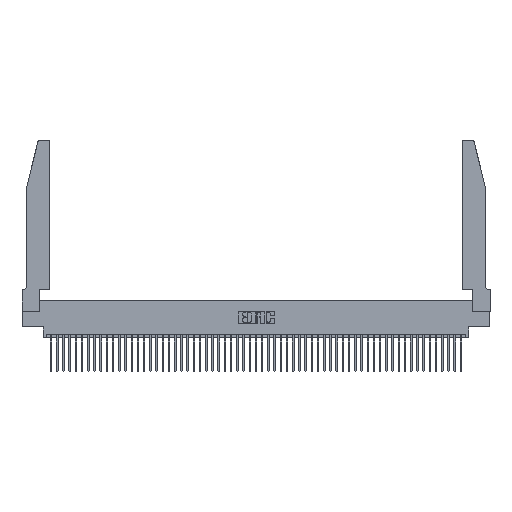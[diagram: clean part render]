
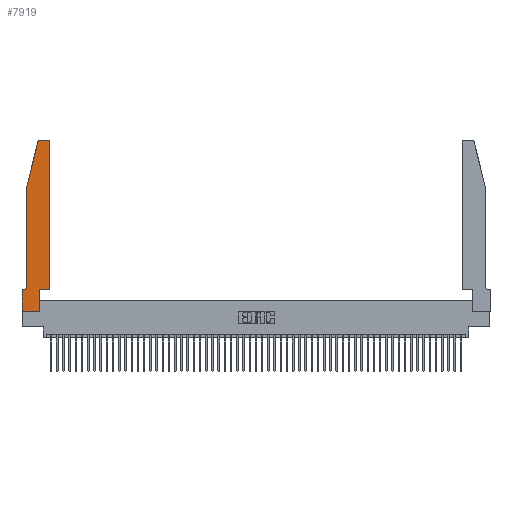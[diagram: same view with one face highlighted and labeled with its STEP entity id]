
A CAD part, top view. The second image highlights one B-rep face of the part: STEP entity #7919.
In plain terms, the highlighted planar face has unit normal (0, 0, 1).
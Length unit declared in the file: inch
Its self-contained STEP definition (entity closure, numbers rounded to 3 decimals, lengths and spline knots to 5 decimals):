
#360 = ORIENTED_EDGE ( 'NONE', *, *, #6956, .T. ) ;
#492 = LINE ( 'NONE', #938, #43675 ) ;
#749 = DIRECTION ( 'NONE',  ( 0., 1., 0. ) ) ;
#938 = CARTESIAN_POINT ( 'NONE',  ( 0.4505, 0.35, 0.37 ) ) ;
#2590 = VECTOR ( 'NONE', #33502, 39.37008 ) ;
#2646 = FACE_OUTER_BOUND ( 'NONE', #4504, .T. ) ;
#3522 = CARTESIAN_POINT ( 'NONE',  ( 0.4205, 2.72, 0.37 ) ) ;
#4024 = DIRECTION ( 'NONE',  ( 0., -1., 0. ) ) ;
#4266 = CARTESIAN_POINT ( 'NONE',  ( 0.0755, 2., 0.37 ) ) ;
#4504 = EDGE_LOOP ( 'NONE', ( #35077, #20084, #11923, #39261, #52693, #35816, #17316, #6054, #360, #19127, #7590, #7361 ) ) ;
#4527 = AXIS2_PLACEMENT_3D ( 'NONE', #27566, #18993, #14943 ) ;
#6054 = ORIENTED_EDGE ( 'NONE', *, *, #8216, .T. ) ;
#6956 = EDGE_CURVE ( 'NONE', #44923, #27076, #21676, .T. ) ;
#7361 = ORIENTED_EDGE ( 'NONE', *, *, #12692, .T. ) ;
#7590 = ORIENTED_EDGE ( 'NONE', *, *, #42156, .T. ) ;
#7919 = ADVANCED_FACE ( 'NONE', ( #2646 ), #35439, .T. ) ;
#8216 = EDGE_CURVE ( 'NONE', #14412, #44923, #12428, .T. ) ;
#8494 = AXIS2_PLACEMENT_3D ( 'NONE', #46907, #8901, #30279 ) ;
#8698 = EDGE_CURVE ( 'NONE', #38435, #44221, #52950, .T. ) ;
#8901 = DIRECTION ( 'NONE',  ( 0., 0., 1. ) ) ;
#11461 = AXIS2_PLACEMENT_3D ( 'NONE', #39875, #18502, #51946 ) ;
#11923 = ORIENTED_EDGE ( 'NONE', *, *, #40419, .T. ) ;
#12428 = LINE ( 'NONE', #50347, #18978 ) ;
#12692 = EDGE_CURVE ( 'NONE', #14862, #17868, #29641, .T. ) ;
#12860 = CARTESIAN_POINT ( 'NONE',  ( 0.2865, 0.35, 0.37 ) ) ;
#14412 = VERTEX_POINT ( 'NONE', #22463 ) ;
#14862 = VERTEX_POINT ( 'NONE', #32825 ) ;
#14943 = DIRECTION ( 'NONE',  ( 1., 0., 0. ) ) ;
#15869 = CARTESIAN_POINT ( 'NONE',  ( 0.0055, 0.35, 0.37 ) ) ;
#16109 = LINE ( 'NONE', #19877, #52101 ) ;
#16722 = CARTESIAN_POINT ( 'NONE',  ( 0.0755, 2., 0.37 ) ) ;
#16853 = DIRECTION ( 'NONE',  ( -1., 0., 0. ) ) ;
#17316 = ORIENTED_EDGE ( 'NONE', *, *, #19793, .T. ) ;
#17868 = VERTEX_POINT ( 'NONE', #32746 ) ;
#18502 = DIRECTION ( 'NONE',  ( 0., 0., -1. ) ) ;
#18978 = VECTOR ( 'NONE', #38453, 39.37008 ) ;
#18993 = DIRECTION ( 'NONE',  ( 0., 0., 1. ) ) ;
#19051 = LINE ( 'NONE', #16722, #51722 ) ;
#19127 = ORIENTED_EDGE ( 'NONE', *, *, #34220, .T. ) ;
#19492 = CARTESIAN_POINT ( 'NONE',  ( 0.4505, 0.35, 0.37 ) ) ;
#19793 = EDGE_CURVE ( 'NONE', #44221, #14412, #50299, .T. ) ;
#19877 = CARTESIAN_POINT ( 'NONE',  ( 0.0755, 2., 0.37 ) ) ;
#20020 = LINE ( 'NONE', #41062, #24580 ) ;
#20084 = ORIENTED_EDGE ( 'NONE', *, *, #39871, .T. ) ;
#20413 = CARTESIAN_POINT ( 'NONE',  ( 0.2865, 0., 0.37 ) ) ;
#21200 = EDGE_CURVE ( 'NONE', #29954, #33107, #16109, .T. ) ;
#21676 = LINE ( 'NONE', #23355, #43976 ) ;
#21954 = VERTEX_POINT ( 'NONE', #28569 ) ;
#22085 = EDGE_CURVE ( 'NONE', #17868, #21954, #35649, .T. ) ;
#22463 = CARTESIAN_POINT ( 'NONE',  ( 0., 0., 0.37 ) ) ;
#23355 = CARTESIAN_POINT ( 'NONE',  ( 0.2865, 0.35, 0.37 ) ) ;
#24565 = CARTESIAN_POINT ( 'NONE',  ( 0., 0.35, 0.37 ) ) ;
#24580 = VECTOR ( 'NONE', #29187, 39.37008 ) ;
#27076 = VERTEX_POINT ( 'NONE', #12860 ) ;
#27566 = CARTESIAN_POINT ( 'NONE',  ( 0., 0.35, 0.37 ) ) ;
#28569 = CARTESIAN_POINT ( 'NONE',  ( 0.284, 2.75, 0.37 ) ) ;
#28717 = CARTESIAN_POINT ( 'NONE',  ( 0.25487, 2.72718, 0.37 ) ) ;
#28938 = CARTESIAN_POINT ( 'NONE',  ( 0.0755, 0.42, 0.37 ) ) ;
#29187 = DIRECTION ( 'NONE',  ( 1., 0., 0. ) ) ;
#29641 = CIRCLE ( 'NONE', #37773, 0.03 ) ;
#29797 = VECTOR ( 'NONE', #16853, 39.37008 ) ;
#29954 = VERTEX_POINT ( 'NONE', #4266 ) ;
#30279 = DIRECTION ( 'NONE',  ( 1., 0., 0. ) ) ;
#32475 = CIRCLE ( 'NONE', #11461, 0.07 ) ;
#32746 = CARTESIAN_POINT ( 'NONE',  ( 0.4205, 2.75, 0.37 ) ) ;
#32763 = DIRECTION ( 'NONE',  ( 0., 0., 1. ) ) ;
#32825 = CARTESIAN_POINT ( 'NONE',  ( 0.4505, 2.72, 0.37 ) ) ;
#33079 = CARTESIAN_POINT ( 'NONE',  ( 0., 0., 0.37 ) ) ;
#33107 = VERTEX_POINT ( 'NONE', #28938 ) ;
#33284 = CARTESIAN_POINT ( 'NONE',  ( 0.2605, 2.75, 0.37 ) ) ;
#33502 = DIRECTION ( 'NONE',  ( -1., 0., 0. ) ) ;
#33506 = EDGE_CURVE ( 'NONE', #33107, #38435, #32475, .T. ) ;
#34220 = EDGE_CURVE ( 'NONE', #27076, #34682, #20020, .T. ) ;
#34682 = VERTEX_POINT ( 'NONE', #19492 ) ;
#35077 = ORIENTED_EDGE ( 'NONE', *, *, #22085, .T. ) ;
#35439 = PLANE ( 'NONE',  #4527 ) ;
#35649 = LINE ( 'NONE', #33284, #29797 ) ;
#35816 = ORIENTED_EDGE ( 'NONE', *, *, #8698, .T. ) ;
#37773 = AXIS2_PLACEMENT_3D ( 'NONE', #3522, #32763, #53792 ) ;
#38045 = CIRCLE ( 'NONE', #8494, 0.03 ) ;
#38435 = VERTEX_POINT ( 'NONE', #15869 ) ;
#38453 = DIRECTION ( 'NONE',  ( 1., 0., 0. ) ) ;
#39261 = ORIENTED_EDGE ( 'NONE', *, *, #21200, .T. ) ;
#39871 = EDGE_CURVE ( 'NONE', #21954, #53599, #38045, .T. ) ;
#39875 = CARTESIAN_POINT ( 'NONE',  ( 0.0055, 0.42, 0.37 ) ) ;
#40419 = EDGE_CURVE ( 'NONE', #53599, #29954, #19051, .T. ) ;
#40678 = DIRECTION ( 'NONE',  ( 0., -1., 0. ) ) ;
#41062 = CARTESIAN_POINT ( 'NONE',  ( 0.4505, 0.35, 0.37 ) ) ;
#42156 = EDGE_CURVE ( 'NONE', #34682, #14862, #492, .T. ) ;
#43675 = VECTOR ( 'NONE', #749, 39.37008 ) ;
#43976 = VECTOR ( 'NONE', #45065, 39.37008 ) ;
#44221 = VERTEX_POINT ( 'NONE', #24565 ) ;
#44923 = VERTEX_POINT ( 'NONE', #20413 ) ;
#45065 = DIRECTION ( 'NONE',  ( 0., 1., 0. ) ) ;
#45596 = DIRECTION ( 'NONE',  ( -0.239, -0.971, 0. ) ) ;
#46907 = CARTESIAN_POINT ( 'NONE',  ( 0.284, 2.72, 0.37 ) ) ;
#49973 = CARTESIAN_POINT ( 'NONE',  ( 0.0755, 0.35, 0.37 ) ) ;
#50299 = LINE ( 'NONE', #33079, #50931 ) ;
#50347 = CARTESIAN_POINT ( 'NONE',  ( 0., 0., 0.37 ) ) ;
#50931 = VECTOR ( 'NONE', #4024, 39.37008 ) ;
#51722 = VECTOR ( 'NONE', #45596, 39.37008 ) ;
#51946 = DIRECTION ( 'NONE',  ( -1., 0., 0. ) ) ;
#52101 = VECTOR ( 'NONE', #40678, 39.37008 ) ;
#52693 = ORIENTED_EDGE ( 'NONE', *, *, #33506, .T. ) ;
#52950 = LINE ( 'NONE', #49973, #2590 ) ;
#53599 = VERTEX_POINT ( 'NONE', #28717 ) ;
#53792 = DIRECTION ( 'NONE',  ( 1., 0., 0. ) ) ;
